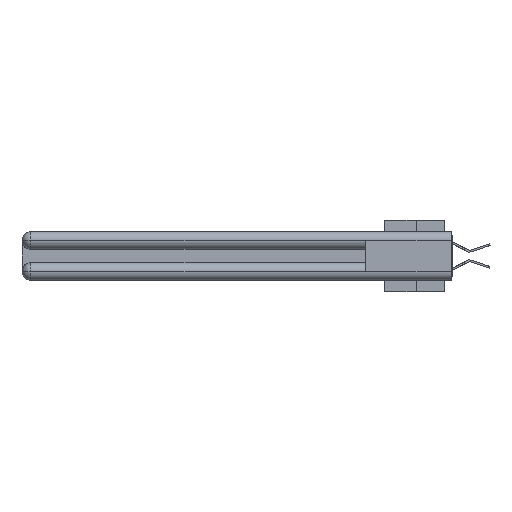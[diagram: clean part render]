
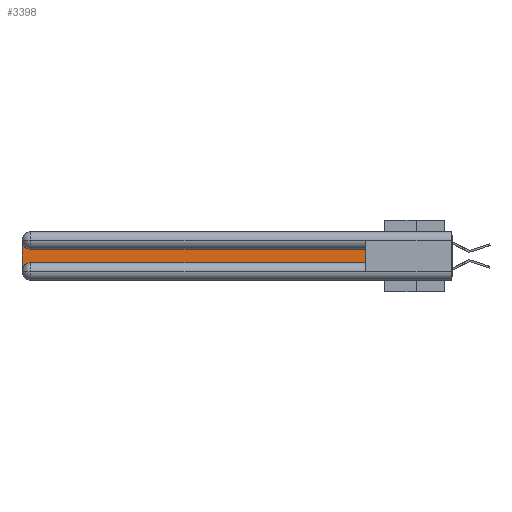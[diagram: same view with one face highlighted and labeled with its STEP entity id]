
A CAD part, left-side view. The second image highlights one B-rep face of the part: STEP entity #3398.
In plain terms, the highlighted planar face has unit normal (-1, 0, 0).
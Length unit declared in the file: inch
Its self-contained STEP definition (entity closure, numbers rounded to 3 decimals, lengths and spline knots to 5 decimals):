
#324 = VERTEX_POINT ( 'NONE', #16387 ) ;
#1552 = EDGE_LOOP ( 'NONE', ( #25957, #28139, #5375, #20461, #16121, #32407 ) ) ;
#1561 = DIRECTION ( 'NONE',  ( 0., 0., -1. ) ) ;
#1935 = CARTESIAN_POINT ( 'NONE',  ( 0.075, 2.94, -0.2175 ) ) ;
#2465 = VERTEX_POINT ( 'NONE', #26909 ) ;
#3013 = CARTESIAN_POINT ( 'NONE',  ( 0.075, 0.6, -0.2175 ) ) ;
#3398 = ADVANCED_FACE ( 'NONE', ( #9759 ), #23743, .F. ) ;
#5375 = ORIENTED_EDGE ( 'NONE', *, *, #28573, .T. ) ;
#6850 = DIRECTION ( 'NONE',  ( 0., 0., -1. ) ) ;
#6990 = LINE ( 'NONE', #18063, #18871 ) ;
#7351 = CARTESIAN_POINT ( 'NONE',  ( 0.075, 0.6, -0.2175 ) ) ;
#8126 = AXIS2_PLACEMENT_3D ( 'NONE', #10276, #15175, #1561 ) ;
#9759 = FACE_OUTER_BOUND ( 'NONE', #1552, .T. ) ;
#9883 = LINE ( 'NONE', #7351, #31220 ) ;
#9953 = EDGE_CURVE ( 'NONE', #324, #2465, #9883, .T. ) ;
#10248 = DIRECTION ( 'NONE',  ( 0., 0., 1. ) ) ;
#10276 = CARTESIAN_POINT ( 'NONE',  ( 0.075, 2.94, -0.0625 ) ) ;
#14808 = LINE ( 'NONE', #3013, #24281 ) ;
#15175 = DIRECTION ( 'NONE',  ( 1., 0., 0. ) ) ;
#15699 = DIRECTION ( 'NONE',  ( 1., 0., 0. ) ) ;
#16121 = ORIENTED_EDGE ( 'NONE', *, *, #26993, .T. ) ;
#16387 = CARTESIAN_POINT ( 'NONE',  ( 0.075, 0.6, -0.2175 ) ) ;
#18063 = CARTESIAN_POINT ( 'NONE',  ( 0.075, 0.6, -0.1225 ) ) ;
#18871 = VECTOR ( 'NONE', #34647, 39.37008 ) ;
#19092 = EDGE_CURVE ( 'NONE', #22058, #25607, #19858, .T. ) ;
#19727 = VECTOR ( 'NONE', #6850, 39.37008 ) ;
#19858 = CIRCLE ( 'NONE', #33905, 0.06 ) ;
#20461 = ORIENTED_EDGE ( 'NONE', *, *, #19092, .T. ) ;
#20648 = CARTESIAN_POINT ( 'NONE',  ( 0.075, 3., -0.2175 ) ) ;
#21281 = CARTESIAN_POINT ( 'NONE',  ( 0.075, 2.94, -0.1225 ) ) ;
#22058 = VERTEX_POINT ( 'NONE', #30956 ) ;
#23704 = VERTEX_POINT ( 'NONE', #21281 ) ;
#23743 = PLANE ( 'NONE',  #25634 ) ;
#23891 = LINE ( 'NONE', #20648, #19727 ) ;
#24281 = VECTOR ( 'NONE', #25550, 39.37008 ) ;
#25550 = DIRECTION ( 'NONE',  ( 0., -1., 0. ) ) ;
#25607 = VERTEX_POINT ( 'NONE', #1935 ) ;
#25634 = AXIS2_PLACEMENT_3D ( 'NONE', #29755, #26112, #34867 ) ;
#25957 = ORIENTED_EDGE ( 'NONE', *, *, #35756, .T. ) ;
#26112 = DIRECTION ( 'NONE',  ( 1., 0., 0. ) ) ;
#26259 = CARTESIAN_POINT ( 'NONE',  ( 0.075, 2.94, -0.2775 ) ) ;
#26909 = CARTESIAN_POINT ( 'NONE',  ( 0.075, 0.6, -0.1225 ) ) ;
#26993 = EDGE_CURVE ( 'NONE', #25607, #324, #14808, .T. ) ;
#28139 = ORIENTED_EDGE ( 'NONE', *, *, #28440, .T. ) ;
#28440 = EDGE_CURVE ( 'NONE', #23704, #35672, #31367, .T. ) ;
#28573 = EDGE_CURVE ( 'NONE', #35672, #22058, #23891, .T. ) ;
#29755 = CARTESIAN_POINT ( 'NONE',  ( 0.075, 3., -0.1225 ) ) ;
#30956 = CARTESIAN_POINT ( 'NONE',  ( 0.075, 3., -0.2775 ) ) ;
#31220 = VECTOR ( 'NONE', #10248, 39.37008 ) ;
#31367 = CIRCLE ( 'NONE', #8126, 0.06 ) ;
#32407 = ORIENTED_EDGE ( 'NONE', *, *, #9953, .T. ) ;
#33905 = AXIS2_PLACEMENT_3D ( 'NONE', #26259, #15699, #35195 ) ;
#34471 = CARTESIAN_POINT ( 'NONE',  ( 0.075, 3., -0.0625 ) ) ;
#34647 = DIRECTION ( 'NONE',  ( 0., 1., 0. ) ) ;
#34867 = DIRECTION ( 'NONE',  ( 0., 0., -1. ) ) ;
#35195 = DIRECTION ( 'NONE',  ( 0., 0., -1. ) ) ;
#35672 = VERTEX_POINT ( 'NONE', #34471 ) ;
#35756 = EDGE_CURVE ( 'NONE', #2465, #23704, #6990, .T. ) ;
